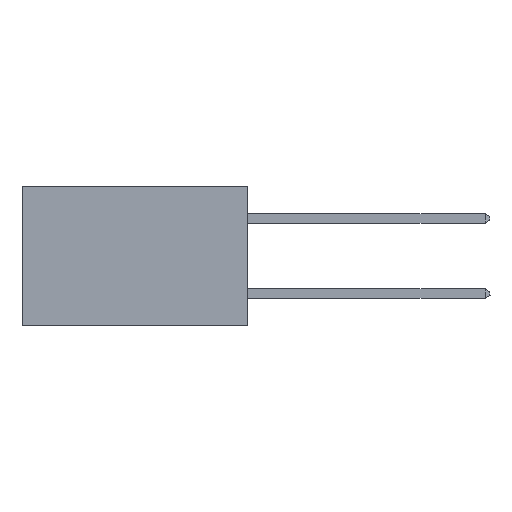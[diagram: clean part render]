
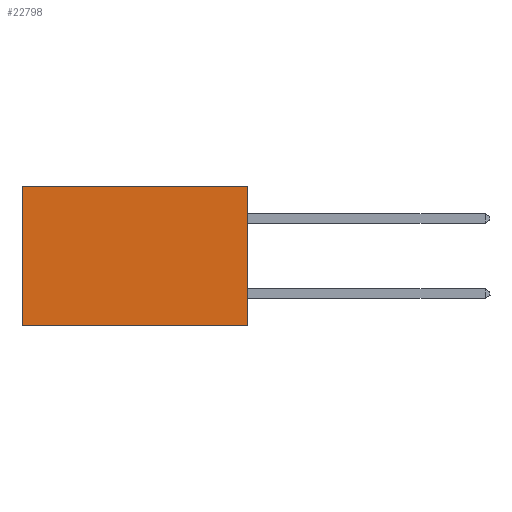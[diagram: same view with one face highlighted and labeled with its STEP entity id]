
A CAD part, left-side view. The second image highlights one B-rep face of the part: STEP entity #22798.
In plain terms, the highlighted planar face has unit normal (-1, 0, 0).
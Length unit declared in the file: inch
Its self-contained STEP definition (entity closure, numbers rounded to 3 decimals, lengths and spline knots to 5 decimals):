
#264 = VECTOR ( 'NONE', #17033, 39.37008 ) ;
#406 = EDGE_CURVE ( 'NONE', #14445, #11322, #22596, .T. ) ;
#988 = CARTESIAN_POINT ( 'NONE',  ( 0.298, 0., -0.37 ) ) ;
#1893 = CARTESIAN_POINT ( 'NONE',  ( 0.298, 0.6, 0. ) ) ;
#2450 = CARTESIAN_POINT ( 'NONE',  ( 0.298, 0.6, -0.37 ) ) ;
#3369 = DIRECTION ( 'NONE',  ( 0., 1., 0. ) ) ;
#4035 = EDGE_CURVE ( 'NONE', #15508, #10974, #18466, .T. ) ;
#4221 = ORIENTED_EDGE ( 'NONE', *, *, #4035, .T. ) ;
#8778 = CARTESIAN_POINT ( 'NONE',  ( 0.298, 0., 0. ) ) ;
#8869 = VECTOR ( 'NONE', #21148, 39.37008 ) ;
#9549 = EDGE_CURVE ( 'NONE', #14445, #15508, #11644, .T. ) ;
#10854 = AXIS2_PLACEMENT_3D ( 'NONE', #26692, #13640, #13442 ) ;
#10974 = VERTEX_POINT ( 'NONE', #2450 ) ;
#11269 = DIRECTION ( 'NONE',  ( 0., 1., 0. ) ) ;
#11322 = VERTEX_POINT ( 'NONE', #23233 ) ;
#11644 = LINE ( 'NONE', #8778, #15722 ) ;
#13264 = ORIENTED_EDGE ( 'NONE', *, *, #406, .F. ) ;
#13442 = DIRECTION ( 'NONE',  ( 0., 0., -1. ) ) ;
#13640 = DIRECTION ( 'NONE',  ( 1., 0., 0. ) ) ;
#14445 = VERTEX_POINT ( 'NONE', #22610 ) ;
#15508 = VERTEX_POINT ( 'NONE', #18347 ) ;
#15722 = VECTOR ( 'NONE', #11269, 39.37008 ) ;
#16160 = VECTOR ( 'NONE', #3369, 39.37008 ) ;
#17033 = DIRECTION ( 'NONE',  ( 0., 0., -1. ) ) ;
#18347 = CARTESIAN_POINT ( 'NONE',  ( 0.298, 0.6, 0. ) ) ;
#18466 = LINE ( 'NONE', #1893, #264 ) ;
#19910 = EDGE_LOOP ( 'NONE', ( #4221, #23384, #13264, #27269 ) ) ;
#21148 = DIRECTION ( 'NONE',  ( 0., 0., -1. ) ) ;
#22596 = LINE ( 'NONE', #23090, #8869 ) ;
#22610 = CARTESIAN_POINT ( 'NONE',  ( 0.298, 0., 0. ) ) ;
#22798 = ADVANCED_FACE ( 'NONE', ( #27962 ), #24472, .F. ) ;
#23090 = CARTESIAN_POINT ( 'NONE',  ( 0.298, 0., 0. ) ) ;
#23233 = CARTESIAN_POINT ( 'NONE',  ( 0.298, 0., -0.37 ) ) ;
#23384 = ORIENTED_EDGE ( 'NONE', *, *, #27194, .F. ) ;
#24472 = PLANE ( 'NONE',  #10854 ) ;
#26471 = LINE ( 'NONE', #988, #16160 ) ;
#26692 = CARTESIAN_POINT ( 'NONE',  ( 0.298, 0., 0. ) ) ;
#27194 = EDGE_CURVE ( 'NONE', #11322, #10974, #26471, .T. ) ;
#27269 = ORIENTED_EDGE ( 'NONE', *, *, #9549, .T. ) ;
#27962 = FACE_OUTER_BOUND ( 'NONE', #19910, .T. ) ;
